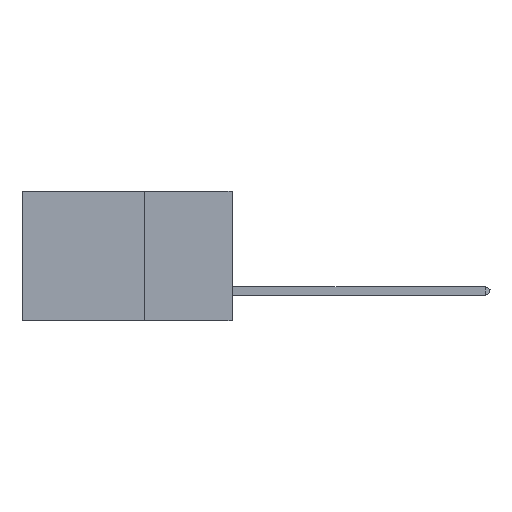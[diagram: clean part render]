
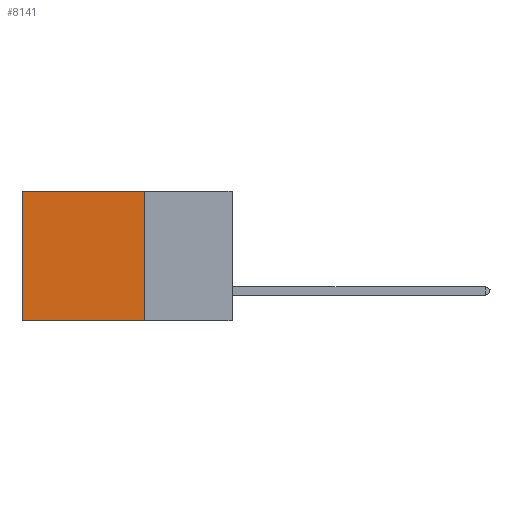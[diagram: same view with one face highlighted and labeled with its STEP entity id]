
A CAD part, left-side view. The second image highlights one B-rep face of the part: STEP entity #8141.
In plain terms, the highlighted planar face has unit normal (-1, 0, 0).
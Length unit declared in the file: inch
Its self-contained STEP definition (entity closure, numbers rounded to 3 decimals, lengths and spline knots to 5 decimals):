
#409 = EDGE_CURVE ( 'NONE', #36334, #32312, #1610, .T. ) ;
#1610 = LINE ( 'NONE', #40079, #10341 ) ;
#4235 = ORIENTED_EDGE ( 'NONE', *, *, #10426, .T. ) ;
#4704 = CARTESIAN_POINT ( 'NONE',  ( 0.2875, 0.25, -0.37 ) ) ;
#4728 = DIRECTION ( 'NONE',  ( 0., 0., -1. ) ) ;
#4835 = DIRECTION ( 'NONE',  ( 0., 1., 0. ) ) ;
#5010 = ORIENTED_EDGE ( 'NONE', *, *, #409, .T. ) ;
#5055 = FACE_OUTER_BOUND ( 'NONE', #31667, .T. ) ;
#8035 = ORIENTED_EDGE ( 'NONE', *, *, #21664, .F. ) ;
#8141 = ADVANCED_FACE ( 'NONE', ( #5055 ), #10712, .F. ) ;
#9943 = VECTOR ( 'NONE', #4835, 39.37008 ) ;
#10341 = VECTOR ( 'NONE', #24209, 39.37008 ) ;
#10426 = EDGE_CURVE ( 'NONE', #35809, #36334, #35495, .T. ) ;
#10517 = EDGE_CURVE ( 'NONE', #36673, #32312, #16189, .T. ) ;
#10712 = PLANE ( 'NONE',  #32052 ) ;
#10849 = DIRECTION ( 'NONE',  ( 1., 0., 0. ) ) ;
#12371 = VECTOR ( 'NONE', #17131, 39.37008 ) ;
#12626 = CARTESIAN_POINT ( 'NONE',  ( 0.2875, 0.6, -0.37 ) ) ;
#16189 = LINE ( 'NONE', #4704, #12371 ) ;
#17032 = CARTESIAN_POINT ( 'NONE',  ( 0.2875, 0.25, 0. ) ) ;
#17131 = DIRECTION ( 'NONE',  ( 0., 1., 0. ) ) ;
#20465 = CARTESIAN_POINT ( 'NONE',  ( 0.2875, 0.25, 0. ) ) ;
#20623 = VECTOR ( 'NONE', #30663, 39.37008 ) ;
#21664 = EDGE_CURVE ( 'NONE', #35809, #36673, #27387, .T. ) ;
#24209 = DIRECTION ( 'NONE',  ( 0., 0., -1. ) ) ;
#27387 = LINE ( 'NONE', #27531, #20623 ) ;
#27531 = CARTESIAN_POINT ( 'NONE',  ( 0.2875, 0.25, 0. ) ) ;
#30663 = DIRECTION ( 'NONE',  ( 0., 0., -1. ) ) ;
#31123 = CARTESIAN_POINT ( 'NONE',  ( 0.2875, 0.25, -0.37 ) ) ;
#31667 = EDGE_LOOP ( 'NONE', ( #5010, #39178, #8035, #4235 ) ) ;
#32052 = AXIS2_PLACEMENT_3D ( 'NONE', #17032, #10849, #4728 ) ;
#32312 = VERTEX_POINT ( 'NONE', #12626 ) ;
#34105 = CARTESIAN_POINT ( 'NONE',  ( 0.2875, 0.6, 0. ) ) ;
#35197 = CARTESIAN_POINT ( 'NONE',  ( 0.2875, 0.25, 0. ) ) ;
#35495 = LINE ( 'NONE', #20465, #9943 ) ;
#35809 = VERTEX_POINT ( 'NONE', #35197 ) ;
#36334 = VERTEX_POINT ( 'NONE', #34105 ) ;
#36673 = VERTEX_POINT ( 'NONE', #31123 ) ;
#39178 = ORIENTED_EDGE ( 'NONE', *, *, #10517, .F. ) ;
#40079 = CARTESIAN_POINT ( 'NONE',  ( 0.2875, 0.6, 0. ) ) ;
